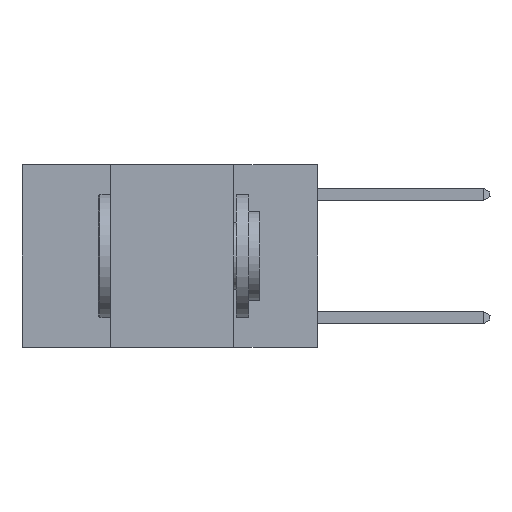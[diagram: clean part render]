
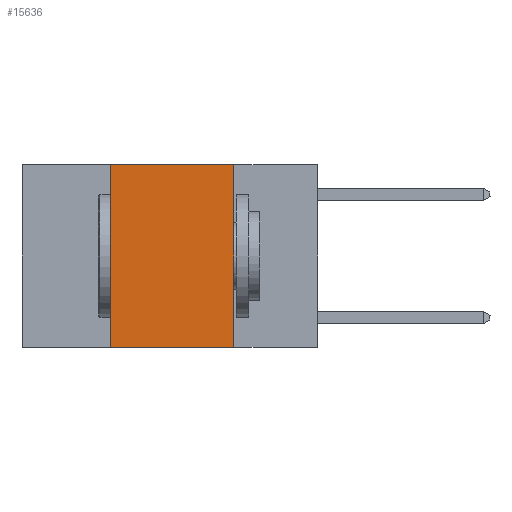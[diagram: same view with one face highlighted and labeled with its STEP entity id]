
A CAD part, left-side view. The second image highlights one B-rep face of the part: STEP entity #15636.
In plain terms, the highlighted planar face has unit normal (-1, 0, 0).
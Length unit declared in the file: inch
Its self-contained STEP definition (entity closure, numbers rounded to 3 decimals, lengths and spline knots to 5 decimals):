
#885 = LINE ( 'NONE', #3672, #25101 ) ;
#893 = EDGE_CURVE ( 'NONE', #15047, #22638, #31771, .T. ) ;
#1111 = ORIENTED_EDGE ( 'NONE', *, *, #2005, .T. ) ;
#1806 = LINE ( 'NONE', #8213, #4100 ) ;
#2005 = EDGE_CURVE ( 'NONE', #18245, #22638, #3219, .T. ) ;
#2886 = CARTESIAN_POINT ( 'NONE',  ( 0., 0.6, -0.37 ) ) ;
#3154 = VERTEX_POINT ( 'NONE', #5179 ) ;
#3219 = LINE ( 'NONE', #2886, #23763 ) ;
#3411 = ORIENTED_EDGE ( 'NONE', *, *, #893, .F. ) ;
#3672 = CARTESIAN_POINT ( 'NONE',  ( 0., 0.6, 0. ) ) ;
#3821 = DIRECTION ( 'NONE',  ( 0., 0., -1. ) ) ;
#4100 = VECTOR ( 'NONE', #13121, 39.37008 ) ;
#5179 = CARTESIAN_POINT ( 'NONE',  ( 0., 0.42, 0. ) ) ;
#6266 = PLANE ( 'NONE',  #22978 ) ;
#8111 = DIRECTION ( 'NONE',  ( 0., -1., 0. ) ) ;
#8213 = CARTESIAN_POINT ( 'NONE',  ( 0., 0.42, 0. ) ) ;
#13121 = DIRECTION ( 'NONE',  ( 0., 0., 1. ) ) ;
#14227 = EDGE_CURVE ( 'NONE', #18245, #3154, #1806, .T. ) ;
#14595 = CARTESIAN_POINT ( 'NONE',  ( 0., 0.17, 0. ) ) ;
#15047 = VERTEX_POINT ( 'NONE', #23156 ) ;
#15541 = ORIENTED_EDGE ( 'NONE', *, *, #14227, .F. ) ;
#15636 = ADVANCED_FACE ( 'NONE', ( #18692 ), #6266, .F. ) ;
#16244 = CARTESIAN_POINT ( 'NONE',  ( 0., 0.6, 0. ) ) ;
#17048 = DIRECTION ( 'NONE',  ( 0., 0., -1. ) ) ;
#17903 = VECTOR ( 'NONE', #17048, 39.37008 ) ;
#18245 = VERTEX_POINT ( 'NONE', #28967 ) ;
#18692 = FACE_OUTER_BOUND ( 'NONE', #32122, .T. ) ;
#22485 = EDGE_CURVE ( 'NONE', #3154, #15047, #885, .T. ) ;
#22638 = VERTEX_POINT ( 'NONE', #28671 ) ;
#22978 = AXIS2_PLACEMENT_3D ( 'NONE', #16244, #26225, #3821 ) ;
#23140 = DIRECTION ( 'NONE',  ( 0., -1., 0. ) ) ;
#23156 = CARTESIAN_POINT ( 'NONE',  ( 0., 0.17, 0. ) ) ;
#23763 = VECTOR ( 'NONE', #8111, 39.37008 ) ;
#24213 = ORIENTED_EDGE ( 'NONE', *, *, #22485, .F. ) ;
#25101 = VECTOR ( 'NONE', #23140, 39.37008 ) ;
#26225 = DIRECTION ( 'NONE',  ( 1., 0., 0. ) ) ;
#28671 = CARTESIAN_POINT ( 'NONE',  ( 0., 0.17, -0.37 ) ) ;
#28967 = CARTESIAN_POINT ( 'NONE',  ( 0., 0.42, -0.37 ) ) ;
#31771 = LINE ( 'NONE', #14595, #17903 ) ;
#32122 = EDGE_LOOP ( 'NONE', ( #3411, #24213, #15541, #1111 ) ) ;
